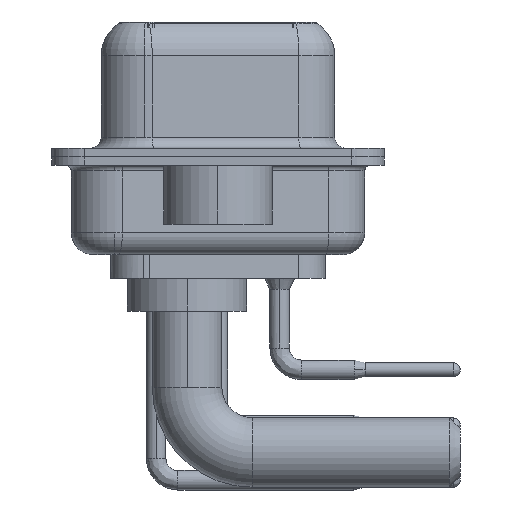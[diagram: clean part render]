
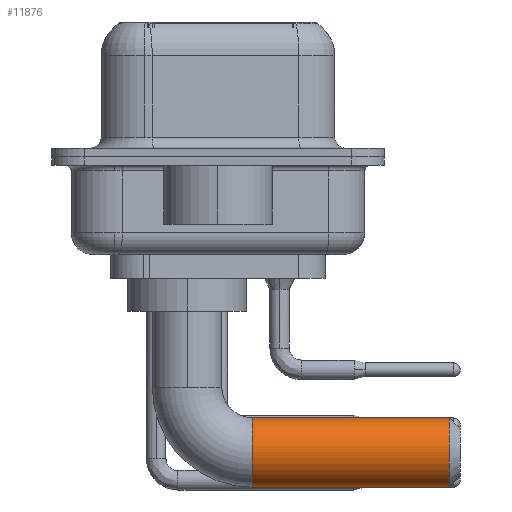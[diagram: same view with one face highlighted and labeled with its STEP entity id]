
A CAD part, left-side view. The second image highlights one B-rep face of the part: STEP entity #11876.
In plain terms, the highlighted cylindrical face has radius 1.6 mm (diameter 3.2 mm), a partial arc.
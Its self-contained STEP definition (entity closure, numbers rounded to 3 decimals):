
#880 = AXIS2_PLACEMENT_3D ( 'NONE', #22329, #25073, #32843 ) ;
#1601 = ORIENTED_EDGE ( 'NONE', *, *, #5551, .T. ) ;
#5490 = EDGE_CURVE ( 'NONE', #18849, #13221, #21752, .T. ) ;
#5551 = EDGE_CURVE ( 'NONE', #13221, #33316, #30234, .T. ) ;
#5764 = AXIS2_PLACEMENT_3D ( 'NONE', #16416, #24686, #14347 ) ;
#5796 = CARTESIAN_POINT ( 'NONE',  ( 0., -12.07, -4.9 ) ) ;
#5865 = DIRECTION ( 'NONE',  ( 0., 0., -1. ) ) ;
#6222 = CARTESIAN_POINT ( 'NONE',  ( 0., -3., -4.9 ) ) ;
#6964 = VECTOR ( 'NONE', #31860, 1000. ) ;
#7612 = AXIS2_PLACEMENT_3D ( 'NONE', #29439, #32198, #5865 ) ;
#8459 = CARTESIAN_POINT ( 'NONE',  ( 0., -3., -4.9 ) ) ;
#9034 = FACE_OUTER_BOUND ( 'NONE', #17172, .T. ) ;
#11876 = ADVANCED_FACE ( 'NONE', ( #9034 ), #32446, .T. ) ;
#13169 = VERTEX_POINT ( 'NONE', #5796 ) ;
#13221 = VERTEX_POINT ( 'NONE', #19289 ) ;
#13367 = CARTESIAN_POINT ( 'NONE',  ( 0., -12.07, -8.1 ) ) ;
#14347 = DIRECTION ( 'NONE',  ( 0., 0., -1. ) ) ;
#14521 = VECTOR ( 'NONE', #32667, 1000. ) ;
#15718 = EDGE_CURVE ( 'NONE', #33316, #13169, #21887, .T. ) ;
#16416 = CARTESIAN_POINT ( 'NONE',  ( 0., -3., -6.5 ) ) ;
#17000 = EDGE_CURVE ( 'NONE', #18849, #13169, #24449, .T. ) ;
#17172 = EDGE_LOOP ( 'NONE', ( #30536, #18814, #1601, #26013 ) ) ;
#18814 = ORIENTED_EDGE ( 'NONE', *, *, #5490, .T. ) ;
#18849 = VERTEX_POINT ( 'NONE', #6222 ) ;
#19289 = CARTESIAN_POINT ( 'NONE',  ( 0., -3., -8.1 ) ) ;
#21752 = CIRCLE ( 'NONE', #880, 1.6 ) ;
#21887 = CIRCLE ( 'NONE', #7612, 1.6 ) ;
#22329 = CARTESIAN_POINT ( 'NONE',  ( 0., -3., -6.5 ) ) ;
#22496 = CARTESIAN_POINT ( 'NONE',  ( 0., -3., -8.1 ) ) ;
#24449 = LINE ( 'NONE', #8459, #6964 ) ;
#24686 = DIRECTION ( 'NONE',  ( 0., -1., 0. ) ) ;
#25073 = DIRECTION ( 'NONE',  ( 0., -1., 0. ) ) ;
#26013 = ORIENTED_EDGE ( 'NONE', *, *, #15718, .T. ) ;
#29439 = CARTESIAN_POINT ( 'NONE',  ( 0., -12.07, -6.5 ) ) ;
#30234 = LINE ( 'NONE', #22496, #14521 ) ;
#30536 = ORIENTED_EDGE ( 'NONE', *, *, #17000, .F. ) ;
#31860 = DIRECTION ( 'NONE',  ( 0., -1., 0. ) ) ;
#32198 = DIRECTION ( 'NONE',  ( 0., 1., 0. ) ) ;
#32446 = CYLINDRICAL_SURFACE ( 'NONE', #5764, 1.6 ) ;
#32667 = DIRECTION ( 'NONE',  ( 0., -1., 0. ) ) ;
#32843 = DIRECTION ( 'NONE',  ( -1., 0., 0. ) ) ;
#33316 = VERTEX_POINT ( 'NONE', #13367 ) ;
